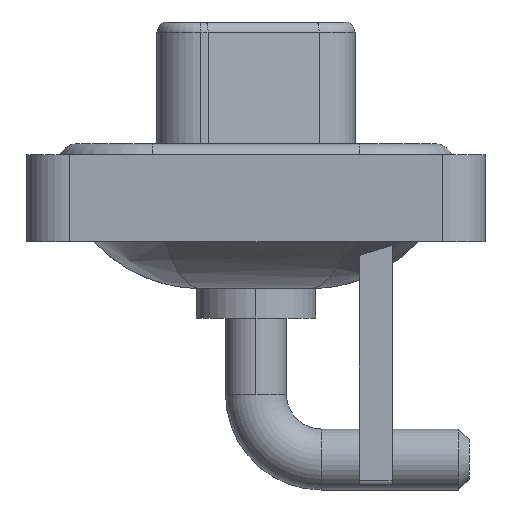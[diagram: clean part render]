
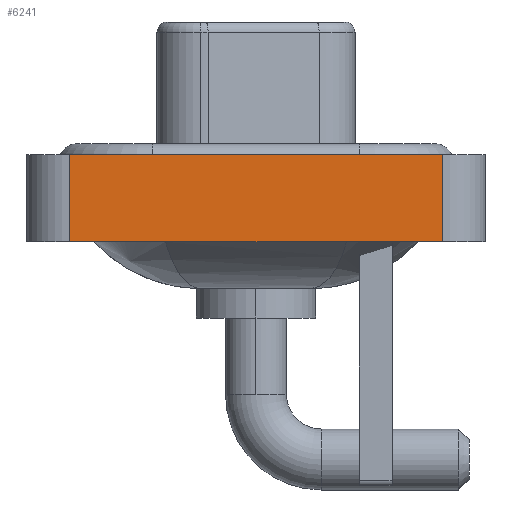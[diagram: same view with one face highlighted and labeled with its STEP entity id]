
A CAD part, left-side view. The second image highlights one B-rep face of the part: STEP entity #6241.
In plain terms, the highlighted planar face has unit normal (-1, 0, 0).
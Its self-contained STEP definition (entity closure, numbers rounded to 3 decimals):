
#856 = DIRECTION ( 'NONE',  ( 0., -1., 0. ) ) ;
#998 = VECTOR ( 'NONE', #10130, 1000. ) ;
#1006 = VERTEX_POINT ( 'NONE', #7842 ) ;
#1077 = VERTEX_POINT ( 'NONE', #13176 ) ;
#1544 = ORIENTED_EDGE ( 'NONE', *, *, #4378, .F. ) ;
#2329 = CARTESIAN_POINT ( 'NONE',  ( -7.3, -8.55, -3.6 ) ) ;
#3819 = DIRECTION ( 'NONE',  ( 0., 0., 1. ) ) ;
#3837 = CARTESIAN_POINT ( 'NONE',  ( -7.3, 8.55, -3.6 ) ) ;
#3971 = CARTESIAN_POINT ( 'NONE',  ( -7.3, -8.55, 0.4 ) ) ;
#4003 = LINE ( 'NONE', #3837, #10227 ) ;
#4295 = EDGE_CURVE ( 'NONE', #16653, #15352, #7240, .T. ) ;
#4378 = EDGE_CURVE ( 'NONE', #1006, #1077, #4003, .T. ) ;
#4605 = LINE ( 'NONE', #11263, #15003 ) ;
#4627 = VECTOR ( 'NONE', #8817, 1000. ) ;
#4795 = LINE ( 'NONE', #11531, #4627 ) ;
#5661 = EDGE_LOOP ( 'NONE', ( #10104, #14798, #1544, #10402 ) ) ;
#6241 = ADVANCED_FACE ( 'NONE', ( #10637 ), #10459, .T. ) ;
#7240 = LINE ( 'NONE', #8641, #998 ) ;
#7842 = CARTESIAN_POINT ( 'NONE',  ( -7.3, 8.55, -3.6 ) ) ;
#8641 = CARTESIAN_POINT ( 'NONE',  ( -7.3, -8.55, -3.6 ) ) ;
#8817 = DIRECTION ( 'NONE',  ( 0., -1., 0. ) ) ;
#9140 = CARTESIAN_POINT ( 'NONE',  ( -7.3, -8.55, -3.6 ) ) ;
#10104 = ORIENTED_EDGE ( 'NONE', *, *, #4295, .T. ) ;
#10130 = DIRECTION ( 'NONE',  ( 0., 0., 1. ) ) ;
#10227 = VECTOR ( 'NONE', #10573, 1000. ) ;
#10402 = ORIENTED_EDGE ( 'NONE', *, *, #14952, .T. ) ;
#10459 = PLANE ( 'NONE',  #16291 ) ;
#10573 = DIRECTION ( 'NONE',  ( 0., 0., 1. ) ) ;
#10637 = FACE_OUTER_BOUND ( 'NONE', #5661, .T. ) ;
#11263 = CARTESIAN_POINT ( 'NONE',  ( -7.3, -8.55, 0.4 ) ) ;
#11531 = CARTESIAN_POINT ( 'NONE',  ( -7.3, -8.55, -3.6 ) ) ;
#13176 = CARTESIAN_POINT ( 'NONE',  ( -7.3, 8.55, 0.4 ) ) ;
#14380 = DIRECTION ( 'NONE',  ( -1., 0., 0. ) ) ;
#14798 = ORIENTED_EDGE ( 'NONE', *, *, #15909, .F. ) ;
#14952 = EDGE_CURVE ( 'NONE', #1006, #16653, #4795, .T. ) ;
#15003 = VECTOR ( 'NONE', #856, 1000. ) ;
#15352 = VERTEX_POINT ( 'NONE', #3971 ) ;
#15909 = EDGE_CURVE ( 'NONE', #1077, #15352, #4605, .T. ) ;
#16291 = AXIS2_PLACEMENT_3D ( 'NONE', #2329, #14380, #3819 ) ;
#16653 = VERTEX_POINT ( 'NONE', #9140 ) ;
